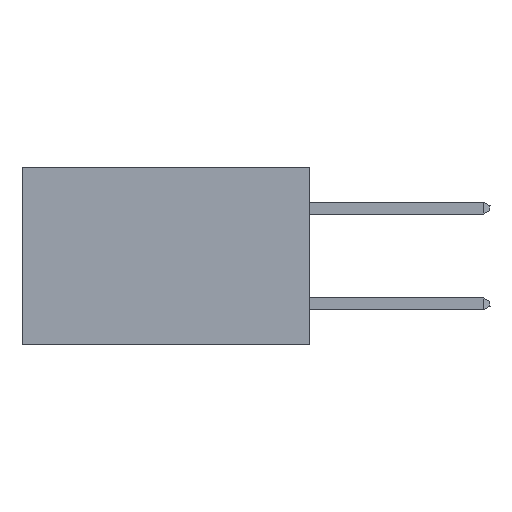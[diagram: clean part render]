
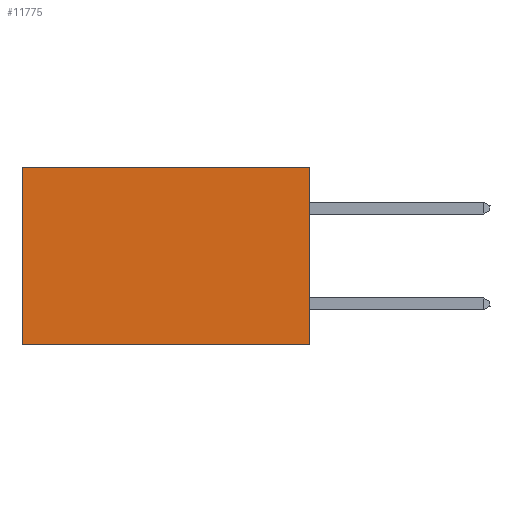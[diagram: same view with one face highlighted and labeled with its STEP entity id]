
A CAD part, left-side view. The second image highlights one B-rep face of the part: STEP entity #11775.
In plain terms, the highlighted planar face has unit normal (-1, 0, 0).
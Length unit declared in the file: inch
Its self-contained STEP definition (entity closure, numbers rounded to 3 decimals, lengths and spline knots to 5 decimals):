
#377 = VERTEX_POINT ( 'NONE', #25563 ) ;
#1371 = FACE_OUTER_BOUND ( 'NONE', #6241, .T. ) ;
#2168 = CARTESIAN_POINT ( 'NONE',  ( 0.2875, 0., 0. ) ) ;
#2323 = PLANE ( 'NONE',  #16330 ) ;
#3249 = DIRECTION ( 'NONE',  ( 0., 0., -1. ) ) ;
#3636 = CARTESIAN_POINT ( 'NONE',  ( 0.2875, 0., -0.37 ) ) ;
#4479 = CARTESIAN_POINT ( 'NONE',  ( 0.2875, 0., 0. ) ) ;
#5070 = ORIENTED_EDGE ( 'NONE', *, *, #18054, .F. ) ;
#6241 = EDGE_LOOP ( 'NONE', ( #24904, #5070, #12975, #11280 ) ) ;
#6726 = VERTEX_POINT ( 'NONE', #26166 ) ;
#7841 = CARTESIAN_POINT ( 'NONE',  ( 0.2875, 0.6, 0. ) ) ;
#9161 = DIRECTION ( 'NONE',  ( 0., 1., 0. ) ) ;
#11063 = LINE ( 'NONE', #2168, #24907 ) ;
#11280 = ORIENTED_EDGE ( 'NONE', *, *, #16245, .T. ) ;
#11775 = ADVANCED_FACE ( 'NONE', ( #1371 ), #2323, .F. ) ;
#12975 = ORIENTED_EDGE ( 'NONE', *, *, #29380, .F. ) ;
#13239 = LINE ( 'NONE', #7841, #28196 ) ;
#13789 = DIRECTION ( 'NONE',  ( 1., 0., 0. ) ) ;
#16163 = VERTEX_POINT ( 'NONE', #24493 ) ;
#16245 = EDGE_CURVE ( 'NONE', #16163, #377, #11063, .T. ) ;
#16330 = AXIS2_PLACEMENT_3D ( 'NONE', #29471, #13789, #24794 ) ;
#17002 = VERTEX_POINT ( 'NONE', #19495 ) ;
#18054 = EDGE_CURVE ( 'NONE', #6726, #17002, #19683, .T. ) ;
#19495 = CARTESIAN_POINT ( 'NONE',  ( 0.2875, 0.6, -0.37 ) ) ;
#19683 = LINE ( 'NONE', #3636, #26218 ) ;
#22622 = EDGE_CURVE ( 'NONE', #377, #17002, #13239, .T. ) ;
#24493 = CARTESIAN_POINT ( 'NONE',  ( 0.2875, 0., 0. ) ) ;
#24794 = DIRECTION ( 'NONE',  ( 0., 0., -1. ) ) ;
#24904 = ORIENTED_EDGE ( 'NONE', *, *, #22622, .T. ) ;
#24907 = VECTOR ( 'NONE', #9161, 39.37008 ) ;
#25563 = CARTESIAN_POINT ( 'NONE',  ( 0.2875, 0.6, 0. ) ) ;
#26166 = CARTESIAN_POINT ( 'NONE',  ( 0.2875, 0., -0.37 ) ) ;
#26218 = VECTOR ( 'NONE', #27004, 39.37008 ) ;
#27004 = DIRECTION ( 'NONE',  ( 0., 1., 0. ) ) ;
#27250 = DIRECTION ( 'NONE',  ( 0., 0., -1. ) ) ;
#27751 = LINE ( 'NONE', #4479, #28866 ) ;
#28196 = VECTOR ( 'NONE', #3249, 39.37008 ) ;
#28866 = VECTOR ( 'NONE', #27250, 39.37008 ) ;
#29380 = EDGE_CURVE ( 'NONE', #16163, #6726, #27751, .T. ) ;
#29471 = CARTESIAN_POINT ( 'NONE',  ( 0.2875, 0., 0. ) ) ;
